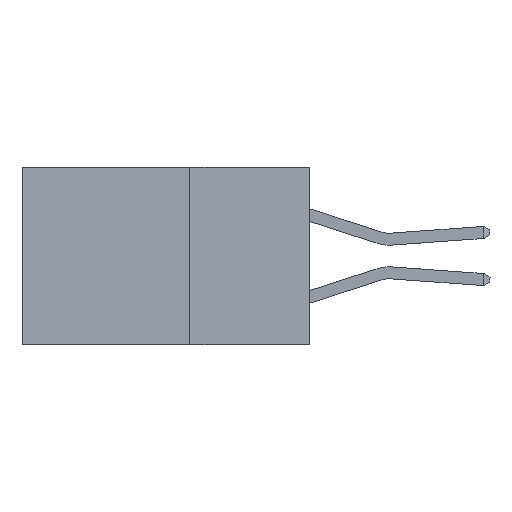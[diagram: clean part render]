
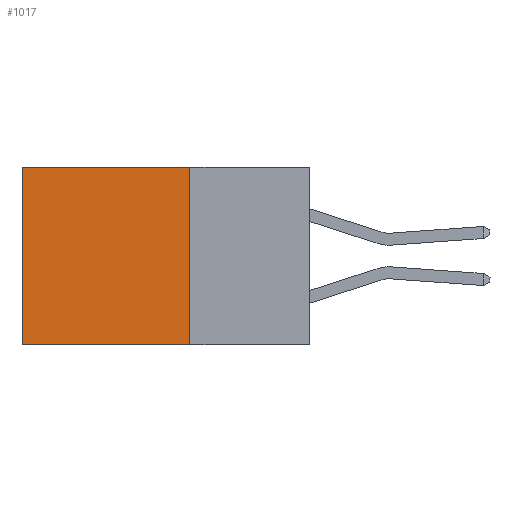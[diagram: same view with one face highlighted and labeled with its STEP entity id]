
A CAD part, left-side view. The second image highlights one B-rep face of the part: STEP entity #1017.
In plain terms, the highlighted planar face has unit normal (-1, 0, 0).
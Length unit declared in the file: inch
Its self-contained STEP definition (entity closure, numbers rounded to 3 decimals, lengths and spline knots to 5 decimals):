
#157 = VERTEX_POINT ( 'NONE', #7397 ) ;
#394 = CARTESIAN_POINT ( 'NONE',  ( 0.298, 0.25, -0.37 ) ) ;
#503 = VECTOR ( 'NONE', #2484, 39.37008 ) ;
#873 = ORIENTED_EDGE ( 'NONE', *, *, #13469, .F. ) ;
#1017 = ADVANCED_FACE ( 'NONE', ( #3518 ), #10731, .F. ) ;
#1277 = ORIENTED_EDGE ( 'NONE', *, *, #14220, .F. ) ;
#1282 = CARTESIAN_POINT ( 'NONE',  ( 0.298, 0.25, 0. ) ) ;
#1353 = VECTOR ( 'NONE', #14098, 39.37008 ) ;
#1447 = CARTESIAN_POINT ( 'NONE',  ( 0.298, 0.25, -0.37 ) ) ;
#1763 = LINE ( 'NONE', #3950, #1353 ) ;
#2021 = VERTEX_POINT ( 'NONE', #2060 ) ;
#2060 = CARTESIAN_POINT ( 'NONE',  ( 0.298, 0.6, -0.37 ) ) ;
#2484 = DIRECTION ( 'NONE',  ( 0., 1., 0. ) ) ;
#3518 = FACE_OUTER_BOUND ( 'NONE', #8109, .T. ) ;
#3950 = CARTESIAN_POINT ( 'NONE',  ( 0.298, 0.6, 0. ) ) ;
#5713 = DIRECTION ( 'NONE',  ( 1., 0., 0. ) ) ;
#6320 = VECTOR ( 'NONE', #16276, 39.37008 ) ;
#7397 = CARTESIAN_POINT ( 'NONE',  ( 0.298, 0.6, 0. ) ) ;
#7400 = ORIENTED_EDGE ( 'NONE', *, *, #12877, .T. ) ;
#7826 = VECTOR ( 'NONE', #11521, 39.37008 ) ;
#8109 = EDGE_LOOP ( 'NONE', ( #7400, #1277, #873, #8602 ) ) ;
#8336 = VERTEX_POINT ( 'NONE', #394 ) ;
#8449 = LINE ( 'NONE', #8526, #6320 ) ;
#8526 = CARTESIAN_POINT ( 'NONE',  ( 0.298, 0.25, 0. ) ) ;
#8602 = ORIENTED_EDGE ( 'NONE', *, *, #14071, .T. ) ;
#8628 = LINE ( 'NONE', #1282, #503 ) ;
#10130 = VERTEX_POINT ( 'NONE', #13546 ) ;
#10731 = PLANE ( 'NONE',  #14151 ) ;
#11521 = DIRECTION ( 'NONE',  ( 0., 1., 0. ) ) ;
#11601 = LINE ( 'NONE', #1447, #7826 ) ;
#12315 = DIRECTION ( 'NONE',  ( 0., 0., -1. ) ) ;
#12877 = EDGE_CURVE ( 'NONE', #157, #2021, #1763, .T. ) ;
#13320 = CARTESIAN_POINT ( 'NONE',  ( 0.298, 0.25, 0. ) ) ;
#13469 = EDGE_CURVE ( 'NONE', #10130, #8336, #8449, .T. ) ;
#13546 = CARTESIAN_POINT ( 'NONE',  ( 0.298, 0.25, 0. ) ) ;
#14071 = EDGE_CURVE ( 'NONE', #10130, #157, #8628, .T. ) ;
#14098 = DIRECTION ( 'NONE',  ( 0., 0., -1. ) ) ;
#14151 = AXIS2_PLACEMENT_3D ( 'NONE', #13320, #5713, #12315 ) ;
#14220 = EDGE_CURVE ( 'NONE', #8336, #2021, #11601, .T. ) ;
#16276 = DIRECTION ( 'NONE',  ( 0., 0., -1. ) ) ;
